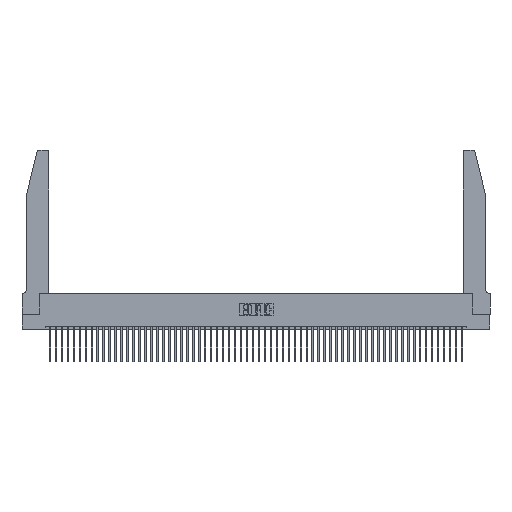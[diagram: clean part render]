
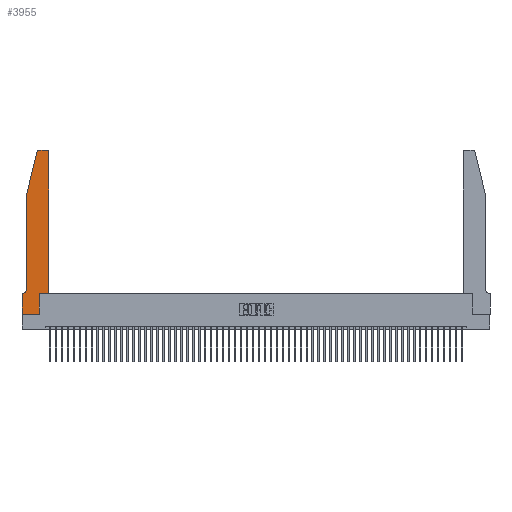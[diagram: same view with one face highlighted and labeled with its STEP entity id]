
A CAD part, top view. The second image highlights one B-rep face of the part: STEP entity #3955.
In plain terms, the highlighted planar face has unit normal (0, 0, 1).
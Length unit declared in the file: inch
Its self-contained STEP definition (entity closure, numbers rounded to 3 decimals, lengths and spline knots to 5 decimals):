
#264 = VERTEX_POINT ( 'NONE', #31185 ) ;
#385 = ORIENTED_EDGE ( 'NONE', *, *, #36658, .T. ) ;
#3376 = CARTESIAN_POINT ( 'NONE',  ( 0.0055, 0.42, 0.37 ) ) ;
#3635 = ORIENTED_EDGE ( 'NONE', *, *, #36964, .T. ) ;
#3955 = ADVANCED_FACE ( 'NONE', ( #42378 ), #25335, .T. ) ;
#4925 = CARTESIAN_POINT ( 'NONE',  ( 0.25487, 2.72718, 0.37 ) ) ;
#6558 = VERTEX_POINT ( 'NONE', #9783 ) ;
#7136 = DIRECTION ( 'NONE',  ( -1., 0., 0. ) ) ;
#7448 = ORIENTED_EDGE ( 'NONE', *, *, #50600, .T. ) ;
#7614 = VECTOR ( 'NONE', #35428, 39.37008 ) ;
#8254 = DIRECTION ( 'NONE',  ( 1., 0., 0. ) ) ;
#8612 = CIRCLE ( 'NONE', #38862, 0.07 ) ;
#8735 = CARTESIAN_POINT ( 'NONE',  ( 0.2865, 0.35, 0.37 ) ) ;
#9783 = CARTESIAN_POINT ( 'NONE',  ( 0.2865, 0., 0.37 ) ) ;
#11142 = EDGE_CURVE ( 'NONE', #20847, #6558, #25149, .T. ) ;
#11993 = CIRCLE ( 'NONE', #52366, 0.03 ) ;
#12099 = CARTESIAN_POINT ( 'NONE',  ( 0., 0.35, 0.37 ) ) ;
#12261 = CARTESIAN_POINT ( 'NONE',  ( 0.284, 2.75, 0.37 ) ) ;
#12755 = CARTESIAN_POINT ( 'NONE',  ( 0.284, 2.72, 0.37 ) ) ;
#13167 = CARTESIAN_POINT ( 'NONE',  ( 0., 0.35, 0.37 ) ) ;
#13617 = VECTOR ( 'NONE', #27291, 39.37008 ) ;
#13837 = CARTESIAN_POINT ( 'NONE',  ( 0.0755, 2., 0.37 ) ) ;
#13876 = VECTOR ( 'NONE', #45661, 39.37008 ) ;
#14181 = DIRECTION ( 'NONE',  ( -1., 0., 0. ) ) ;
#14863 = VERTEX_POINT ( 'NONE', #51622 ) ;
#15304 = LINE ( 'NONE', #48080, #34266 ) ;
#15579 = VERTEX_POINT ( 'NONE', #22668 ) ;
#16019 = ORIENTED_EDGE ( 'NONE', *, *, #38085, .T. ) ;
#16580 = CARTESIAN_POINT ( 'NONE',  ( 0.4505, 0.35, 0.37 ) ) ;
#16713 = ORIENTED_EDGE ( 'NONE', *, *, #11142, .T. ) ;
#17478 = DIRECTION ( 'NONE',  ( 1., 0., 0. ) ) ;
#18359 = CARTESIAN_POINT ( 'NONE',  ( 0.0755, 0.35, 0.37 ) ) ;
#19516 = DIRECTION ( 'NONE',  ( -1., 0., 0. ) ) ;
#20328 = DIRECTION ( 'NONE',  ( 0., 0., -1. ) ) ;
#20762 = DIRECTION ( 'NONE',  ( 1., 0., 0. ) ) ;
#20783 = DIRECTION ( 'NONE',  ( 0., 0., 1. ) ) ;
#20847 = VERTEX_POINT ( 'NONE', #20941 ) ;
#20873 = ORIENTED_EDGE ( 'NONE', *, *, #51485, .T. ) ;
#20941 = CARTESIAN_POINT ( 'NONE',  ( 0., 0., 0.37 ) ) ;
#22420 = DIRECTION ( 'NONE',  ( 0., 1., 0. ) ) ;
#22527 = ORIENTED_EDGE ( 'NONE', *, *, #39037, .T. ) ;
#22668 = CARTESIAN_POINT ( 'NONE',  ( 0.4205, 2.75, 0.37 ) ) ;
#23081 = VERTEX_POINT ( 'NONE', #4925 ) ;
#23618 = ORIENTED_EDGE ( 'NONE', *, *, #29899, .T. ) ;
#24059 = CIRCLE ( 'NONE', #42964, 0.03 ) ;
#24510 = CARTESIAN_POINT ( 'NONE',  ( 0.0055, 0.35, 0.37 ) ) ;
#24784 = CARTESIAN_POINT ( 'NONE',  ( 0.0755, 2., 0.37 ) ) ;
#25149 = LINE ( 'NONE', #48844, #13617 ) ;
#25335 = PLANE ( 'NONE',  #32729 ) ;
#25700 = LINE ( 'NONE', #16580, #51388 ) ;
#26012 = DIRECTION ( 'NONE',  ( 0., 0., 1. ) ) ;
#26760 = LINE ( 'NONE', #37339, #13876 ) ;
#27291 = DIRECTION ( 'NONE',  ( 1., 0., 0. ) ) ;
#27518 = DIRECTION ( 'NONE',  ( 0., 1., 0. ) ) ;
#29899 = EDGE_CURVE ( 'NONE', #51087, #20847, #37682, .T. ) ;
#31185 = CARTESIAN_POINT ( 'NONE',  ( 0.0755, 0.42, 0.37 ) ) ;
#31799 = ORIENTED_EDGE ( 'NONE', *, *, #46898, .T. ) ;
#32512 = VECTOR ( 'NONE', #27518, 39.37008 ) ;
#32729 = AXIS2_PLACEMENT_3D ( 'NONE', #12099, #20783, #42284 ) ;
#33168 = VERTEX_POINT ( 'NONE', #8735 ) ;
#34266 = VECTOR ( 'NONE', #22420, 39.37008 ) ;
#35428 = DIRECTION ( 'NONE',  ( 0., -1., 0. ) ) ;
#35671 = VECTOR ( 'NONE', #14181, 39.37008 ) ;
#36360 = VECTOR ( 'NONE', #50093, 39.37008 ) ;
#36658 = EDGE_CURVE ( 'NONE', #55686, #264, #42760, .T. ) ;
#36912 = VERTEX_POINT ( 'NONE', #46132 ) ;
#36964 = EDGE_CURVE ( 'NONE', #15579, #46078, #44097, .T. ) ;
#37053 = CARTESIAN_POINT ( 'NONE',  ( 0., 0., 0.37 ) ) ;
#37339 = CARTESIAN_POINT ( 'NONE',  ( 0.0755, 2., 0.37 ) ) ;
#37682 = LINE ( 'NONE', #37053, #36360 ) ;
#38085 = EDGE_CURVE ( 'NONE', #6558, #33168, #44630, .T. ) ;
#38293 = CARTESIAN_POINT ( 'NONE',  ( 0.4205, 2.72, 0.37 ) ) ;
#38862 = AXIS2_PLACEMENT_3D ( 'NONE', #3376, #20328, #7136 ) ;
#39037 = EDGE_CURVE ( 'NONE', #33168, #14863, #25700, .T. ) ;
#39992 = CARTESIAN_POINT ( 'NONE',  ( 0.2865, 0.35, 0.37 ) ) ;
#40481 = EDGE_LOOP ( 'NONE', ( #3635, #52185, #20873, #385, #49241, #7448, #23618, #16713, #16019, #22527, #31799, #53445 ) ) ;
#42284 = DIRECTION ( 'NONE',  ( 1., 0., 0. ) ) ;
#42378 = FACE_OUTER_BOUND ( 'NONE', #40481, .T. ) ;
#42514 = VERTEX_POINT ( 'NONE', #24510 ) ;
#42760 = LINE ( 'NONE', #13837, #7614 ) ;
#42964 = AXIS2_PLACEMENT_3D ( 'NONE', #12755, #55338, #8254 ) ;
#44097 = LINE ( 'NONE', #45398, #48832 ) ;
#44630 = LINE ( 'NONE', #39992, #32512 ) ;
#45398 = CARTESIAN_POINT ( 'NONE',  ( 0.2605, 2.75, 0.37 ) ) ;
#45661 = DIRECTION ( 'NONE',  ( -0.239, -0.971, 0. ) ) ;
#46078 = VERTEX_POINT ( 'NONE', #12261 ) ;
#46132 = CARTESIAN_POINT ( 'NONE',  ( 0.4505, 2.72, 0.37 ) ) ;
#46619 = EDGE_CURVE ( 'NONE', #264, #42514, #8612, .T. ) ;
#46898 = EDGE_CURVE ( 'NONE', #14863, #36912, #15304, .T. ) ;
#48080 = CARTESIAN_POINT ( 'NONE',  ( 0.4505, 0.35, 0.37 ) ) ;
#48832 = VECTOR ( 'NONE', #19516, 39.37008 ) ;
#48844 = CARTESIAN_POINT ( 'NONE',  ( 0., 0., 0.37 ) ) ;
#49241 = ORIENTED_EDGE ( 'NONE', *, *, #46619, .T. ) ;
#49720 = EDGE_CURVE ( 'NONE', #36912, #15579, #11993, .T. ) ;
#50093 = DIRECTION ( 'NONE',  ( 0., -1., 0. ) ) ;
#50600 = EDGE_CURVE ( 'NONE', #42514, #51087, #51867, .T. ) ;
#51087 = VERTEX_POINT ( 'NONE', #13167 ) ;
#51388 = VECTOR ( 'NONE', #20762, 39.37008 ) ;
#51485 = EDGE_CURVE ( 'NONE', #23081, #55686, #26760, .T. ) ;
#51550 = EDGE_CURVE ( 'NONE', #46078, #23081, #24059, .T. ) ;
#51622 = CARTESIAN_POINT ( 'NONE',  ( 0.4505, 0.35, 0.37 ) ) ;
#51867 = LINE ( 'NONE', #18359, #35671 ) ;
#52185 = ORIENTED_EDGE ( 'NONE', *, *, #51550, .T. ) ;
#52366 = AXIS2_PLACEMENT_3D ( 'NONE', #38293, #26012, #17478 ) ;
#53445 = ORIENTED_EDGE ( 'NONE', *, *, #49720, .T. ) ;
#55338 = DIRECTION ( 'NONE',  ( 0., 0., 1. ) ) ;
#55686 = VERTEX_POINT ( 'NONE', #24784 ) ;
